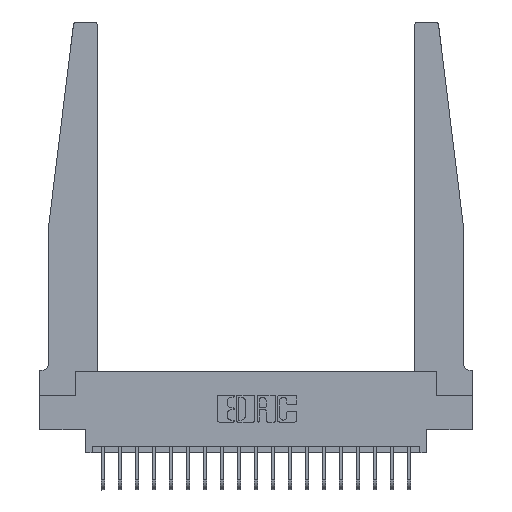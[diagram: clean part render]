
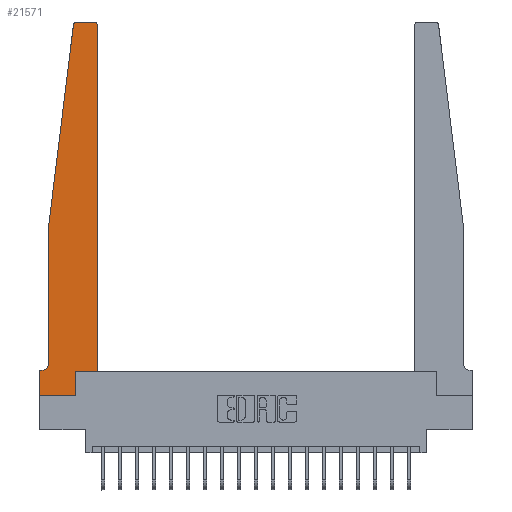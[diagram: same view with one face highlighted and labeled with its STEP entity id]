
A CAD part, top view. The second image highlights one B-rep face of the part: STEP entity #21571.
In plain terms, the highlighted planar face has unit normal (0, 0, 1).
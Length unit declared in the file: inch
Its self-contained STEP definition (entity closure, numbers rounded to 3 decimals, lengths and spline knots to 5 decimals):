
#141 = DIRECTION ( 'NONE',  ( -1., 0., 0. ) ) ;
#205 = DIRECTION ( 'NONE',  ( -0.122, -0.992, 0. ) ) ;
#946 = EDGE_CURVE ( 'NONE', #10975, #11932, #12458, .T. ) ;
#1084 = VERTEX_POINT ( 'NONE', #13943 ) ;
#1811 = EDGE_CURVE ( 'NONE', #20020, #18568, #14128, .T. ) ;
#1929 = VECTOR ( 'NONE', #10058, 39.37008 ) ;
#2188 = DIRECTION ( 'NONE',  ( 0., 0., 1. ) ) ;
#2195 = CARTESIAN_POINT ( 'NONE',  ( 0.2605, 0.18, 0.37 ) ) ;
#2301 = LINE ( 'NONE', #12947, #2671 ) ;
#2434 = VERTEX_POINT ( 'NONE', #15083 ) ;
#2453 = LINE ( 'NONE', #4289, #9748 ) ;
#2544 = ORIENTED_EDGE ( 'NONE', *, *, #5759, .T. ) ;
#2633 = VECTOR ( 'NONE', #15902, 39.37008 ) ;
#2671 = VECTOR ( 'NONE', #9268, 39.37008 ) ;
#3097 = CIRCLE ( 'NONE', #18058, 0.03 ) ;
#3142 = CARTESIAN_POINT ( 'NONE',  ( 0.425, 0.18, 0.37 ) ) ;
#3334 = EDGE_CURVE ( 'NONE', #10212, #12622, #2453, .T. ) ;
#3340 = CARTESIAN_POINT ( 'NONE',  ( 0.2605, 0., 0.37 ) ) ;
#3410 = ORIENTED_EDGE ( 'NONE', *, *, #6642, .T. ) ;
#3717 = DIRECTION ( 'NONE',  ( 0., -1., 0. ) ) ;
#3831 = EDGE_CURVE ( 'NONE', #15268, #18195, #13399, .T. ) ;
#4069 = ORIENTED_EDGE ( 'NONE', *, *, #21598, .T. ) ;
#4213 = EDGE_CURVE ( 'NONE', #1084, #10975, #3097, .T. ) ;
#4289 = CARTESIAN_POINT ( 'NONE',  ( 0., 0., 0.37 ) ) ;
#4857 = AXIS2_PLACEMENT_3D ( 'NONE', #19447, #2188, #14661 ) ;
#5448 = CARTESIAN_POINT ( 'NONE',  ( 0.065, 1.25, 0.37 ) ) ;
#5482 = ORIENTED_EDGE ( 'NONE', *, *, #13660, .T. ) ;
#5759 = EDGE_CURVE ( 'NONE', #2434, #10212, #22497, .T. ) ;
#6642 = EDGE_CURVE ( 'NONE', #18195, #20020, #16327, .T. ) ;
#6883 = VERTEX_POINT ( 'NONE', #18934 ) ;
#6909 = VERTEX_POINT ( 'NONE', #19269 ) ;
#7474 = CARTESIAN_POINT ( 'NONE',  ( 0., 0., 0.37 ) ) ;
#7487 = DIRECTION ( 'NONE',  ( 1., 0., 0. ) ) ;
#7681 = ORIENTED_EDGE ( 'NONE', *, *, #4213, .T. ) ;
#7833 = ORIENTED_EDGE ( 'NONE', *, *, #946, .T. ) ;
#8234 = DIRECTION ( 'NONE',  ( 1., 0., 0. ) ) ;
#9268 = DIRECTION ( 'NONE',  ( -1., 0., 0. ) ) ;
#9418 = DIRECTION ( 'NONE',  ( 0., 0., 1. ) ) ;
#9748 = VECTOR ( 'NONE', #7487, 39.37008 ) ;
#10058 = DIRECTION ( 'NONE',  ( 0., 1., 0. ) ) ;
#10212 = VERTEX_POINT ( 'NONE', #7474 ) ;
#10578 = CARTESIAN_POINT ( 'NONE',  ( 0., 0., 0.37 ) ) ;
#10649 = CARTESIAN_POINT ( 'NONE',  ( 0.25, 2.75, 0.37 ) ) ;
#10975 = VERTEX_POINT ( 'NONE', #17599 ) ;
#11002 = VECTOR ( 'NONE', #8234, 39.37008 ) ;
#11243 = AXIS2_PLACEMENT_3D ( 'NONE', #11741, #15047, #15159 ) ;
#11480 = DIRECTION ( 'NONE',  ( 1., 0., 0. ) ) ;
#11614 = LINE ( 'NONE', #10649, #2633 ) ;
#11741 = CARTESIAN_POINT ( 'NONE',  ( 0.395, 2.72, 0.37 ) ) ;
#11932 = VERTEX_POINT ( 'NONE', #20300 ) ;
#12394 = ORIENTED_EDGE ( 'NONE', *, *, #16646, .T. ) ;
#12458 = LINE ( 'NONE', #15876, #19000 ) ;
#12622 = VERTEX_POINT ( 'NONE', #3340 ) ;
#12947 = CARTESIAN_POINT ( 'NONE',  ( 0.065, 0.1875, 0.37 ) ) ;
#13399 = LINE ( 'NONE', #18977, #11002 ) ;
#13660 = EDGE_CURVE ( 'NONE', #6909, #6883, #15858, .T. ) ;
#13770 = ORIENTED_EDGE ( 'NONE', *, *, #16962, .T. ) ;
#13943 = CARTESIAN_POINT ( 'NONE',  ( 0.27653, 2.75, 0.37 ) ) ;
#14128 = CIRCLE ( 'NONE', #11243, 0.03 ) ;
#14427 = PLANE ( 'NONE',  #4857 ) ;
#14458 = DIRECTION ( 'NONE',  ( 0., 0., -1. ) ) ;
#14571 = CARTESIAN_POINT ( 'NONE',  ( 0.015, 0.2375, 0.37 ) ) ;
#14661 = DIRECTION ( 'NONE',  ( 1., 0., 0. ) ) ;
#14795 = CARTESIAN_POINT ( 'NONE',  ( 0.425, 2.72, 0.37 ) ) ;
#14959 = AXIS2_PLACEMENT_3D ( 'NONE', #14571, #14458, #141 ) ;
#15047 = DIRECTION ( 'NONE',  ( 0., 0., 1. ) ) ;
#15083 = CARTESIAN_POINT ( 'NONE',  ( 0., 0.1875, 0.37 ) ) ;
#15159 = DIRECTION ( 'NONE',  ( 1., 0., 0. ) ) ;
#15268 = VERTEX_POINT ( 'NONE', #2195 ) ;
#15425 = LINE ( 'NONE', #22426, #1929 ) ;
#15858 = CIRCLE ( 'NONE', #14959, 0.05 ) ;
#15876 = CARTESIAN_POINT ( 'NONE',  ( 0.065, 1.25, 0.37 ) ) ;
#15902 = DIRECTION ( 'NONE',  ( -1., 0., 0. ) ) ;
#16207 = CARTESIAN_POINT ( 'NONE',  ( 0.425, 0.18, 0.37 ) ) ;
#16327 = LINE ( 'NONE', #16207, #21369 ) ;
#16583 = ORIENTED_EDGE ( 'NONE', *, *, #17398, .T. ) ;
#16646 = EDGE_CURVE ( 'NONE', #11932, #6909, #21339, .T. ) ;
#16884 = VECTOR ( 'NONE', #3717, 39.37008 ) ;
#16962 = EDGE_CURVE ( 'NONE', #18568, #1084, #11614, .T. ) ;
#17066 = CARTESIAN_POINT ( 'NONE',  ( 0.395, 2.75, 0.37 ) ) ;
#17398 = EDGE_CURVE ( 'NONE', #12622, #15268, #15425, .T. ) ;
#17599 = CARTESIAN_POINT ( 'NONE',  ( 0.24675, 2.72367, 0.37 ) ) ;
#17957 = FACE_OUTER_BOUND ( 'NONE', #21969, .T. ) ;
#18058 = AXIS2_PLACEMENT_3D ( 'NONE', #19708, #9418, #11480 ) ;
#18145 = DIRECTION ( 'NONE',  ( 0., 1., 0. ) ) ;
#18195 = VERTEX_POINT ( 'NONE', #3142 ) ;
#18568 = VERTEX_POINT ( 'NONE', #17066 ) ;
#18744 = ORIENTED_EDGE ( 'NONE', *, *, #3831, .T. ) ;
#18934 = CARTESIAN_POINT ( 'NONE',  ( 0.015, 0.1875, 0.37 ) ) ;
#18977 = CARTESIAN_POINT ( 'NONE',  ( 0.425, 0.18, 0.37 ) ) ;
#19000 = VECTOR ( 'NONE', #205, 39.37008 ) ;
#19043 = DIRECTION ( 'NONE',  ( 0., -1., 0. ) ) ;
#19269 = CARTESIAN_POINT ( 'NONE',  ( 0.065, 0.2375, 0.37 ) ) ;
#19447 = CARTESIAN_POINT ( 'NONE',  ( 0., 0.1875, 0.37 ) ) ;
#19708 = CARTESIAN_POINT ( 'NONE',  ( 0.27653, 2.72, 0.37 ) ) ;
#19720 = ORIENTED_EDGE ( 'NONE', *, *, #3334, .T. ) ;
#19837 = ORIENTED_EDGE ( 'NONE', *, *, #1811, .T. ) ;
#20020 = VERTEX_POINT ( 'NONE', #14795 ) ;
#20300 = CARTESIAN_POINT ( 'NONE',  ( 0.065, 1.25, 0.37 ) ) ;
#20994 = VECTOR ( 'NONE', #19043, 39.37008 ) ;
#21339 = LINE ( 'NONE', #5448, #16884 ) ;
#21369 = VECTOR ( 'NONE', #18145, 39.37008 ) ;
#21571 = ADVANCED_FACE ( 'NONE', ( #17957 ), #14427, .T. ) ;
#21598 = EDGE_CURVE ( 'NONE', #6883, #2434, #2301, .T. ) ;
#21969 = EDGE_LOOP ( 'NONE', ( #13770, #7681, #7833, #12394, #5482, #4069, #2544, #19720, #16583, #18744, #3410, #19837 ) ) ;
#22426 = CARTESIAN_POINT ( 'NONE',  ( 0.2605, 0.18, 0.37 ) ) ;
#22497 = LINE ( 'NONE', #10578, #20994 ) ;
